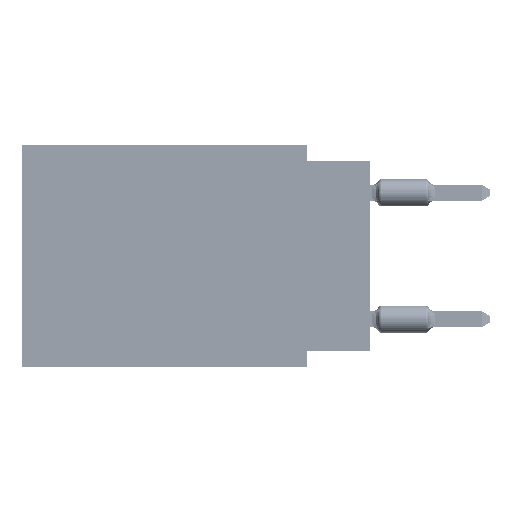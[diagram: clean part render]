
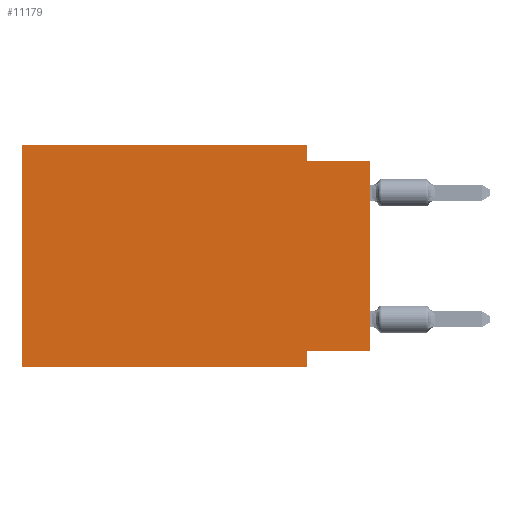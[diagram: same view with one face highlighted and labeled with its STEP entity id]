
A CAD part, left-side view. The second image highlights one B-rep face of the part: STEP entity #11179.
In plain terms, the highlighted planar face has unit normal (-1, 0, 0).
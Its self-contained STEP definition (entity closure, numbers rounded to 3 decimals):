
#1125 = CARTESIAN_POINT ( 'NONE',  ( 0., 0., -8.255 ) ) ;
#1972 = LINE ( 'NONE', #7984, #21266 ) ;
#5034 = EDGE_CURVE ( 'NONE', #32759, #79217, #30150, .T. ) ;
#5221 = CARTESIAN_POINT ( 'NONE',  ( 0., 2.54, 0. ) ) ;
#5799 = DIRECTION ( 'NONE',  ( 0., 0., 1. ) ) ;
#7984 = CARTESIAN_POINT ( 'NONE',  ( 0., 2.54, 0. ) ) ;
#10133 = VECTOR ( 'NONE', #76209, 1000. ) ;
#11179 = ADVANCED_FACE ( 'NONE', ( #45093 ), #71273, .F. ) ;
#11938 = CARTESIAN_POINT ( 'NONE',  ( 0., 0., -0.635 ) ) ;
#12740 = DIRECTION ( 'NONE',  ( 0., 1., 0. ) ) ;
#12816 = DIRECTION ( 'NONE',  ( 0., -1., 0. ) ) ;
#16610 = EDGE_CURVE ( 'NONE', #21372, #56353, #16953, .T. ) ;
#16953 = LINE ( 'NONE', #37131, #10133 ) ;
#17264 = DIRECTION ( 'NONE',  ( 0., -1., 0. ) ) ;
#17444 = CARTESIAN_POINT ( 'NONE',  ( 0., 13.97, 0. ) ) ;
#17733 = EDGE_CURVE ( 'NONE', #38163, #23053, #1972, .T. ) ;
#18718 = LINE ( 'NONE', #17444, #49562 ) ;
#21266 = VECTOR ( 'NONE', #40644, 1000. ) ;
#21372 = VERTEX_POINT ( 'NONE', #33781 ) ;
#23053 = VERTEX_POINT ( 'NONE', #28946 ) ;
#26891 = ORIENTED_EDGE ( 'NONE', *, *, #17733, .F. ) ;
#28946 = CARTESIAN_POINT ( 'NONE',  ( 0., 2.54, -0.635 ) ) ;
#29073 = ORIENTED_EDGE ( 'NONE', *, *, #5034, .T. ) ;
#29347 = AXIS2_PLACEMENT_3D ( 'NONE', #34309, #33896, #41602 ) ;
#29503 = EDGE_LOOP ( 'NONE', ( #34919, #46568, #26891, #70943, #56442, #29073, #61359, #41374 ) ) ;
#30150 = LINE ( 'NONE', #31843, #45351 ) ;
#30372 = EDGE_CURVE ( 'NONE', #21372, #83384, #59988, .T. ) ;
#31843 = CARTESIAN_POINT ( 'NONE',  ( 0., 13.97, -8.89 ) ) ;
#32759 = VERTEX_POINT ( 'NONE', #78496 ) ;
#33781 = CARTESIAN_POINT ( 'NONE',  ( 0., 0., -8.255 ) ) ;
#33896 = DIRECTION ( 'NONE',  ( 1., 0., 0. ) ) ;
#34309 = CARTESIAN_POINT ( 'NONE',  ( 0., 13.97, 0. ) ) ;
#34633 = VERTEX_POINT ( 'NONE', #61239 ) ;
#34919 = ORIENTED_EDGE ( 'NONE', *, *, #16610, .T. ) ;
#37131 = CARTESIAN_POINT ( 'NONE',  ( 0., 0., 0. ) ) ;
#38163 = VERTEX_POINT ( 'NONE', #5221 ) ;
#40644 = DIRECTION ( 'NONE',  ( 0., 0., -1. ) ) ;
#41374 = ORIENTED_EDGE ( 'NONE', *, *, #30372, .F. ) ;
#41602 = DIRECTION ( 'NONE',  ( 0., 0., -1. ) ) ;
#45093 = FACE_OUTER_BOUND ( 'NONE', #29503, .T. ) ;
#45116 = CARTESIAN_POINT ( 'NONE',  ( 0., 2.54, -8.89 ) ) ;
#45167 = VECTOR ( 'NONE', #12740, 1000. ) ;
#45351 = VECTOR ( 'NONE', #17264, 1000. ) ;
#46568 = ORIENTED_EDGE ( 'NONE', *, *, #63101, .F. ) ;
#49562 = VECTOR ( 'NONE', #5799, 1000. ) ;
#49783 = VECTOR ( 'NONE', #69328, 1000. ) ;
#51070 = CARTESIAN_POINT ( 'NONE',  ( 0., 0., -0.635 ) ) ;
#52403 = EDGE_CURVE ( 'NONE', #32759, #34633, #18718, .T. ) ;
#55951 = EDGE_CURVE ( 'NONE', #83384, #79217, #77733, .T. ) ;
#56353 = VERTEX_POINT ( 'NONE', #11938 ) ;
#56442 = ORIENTED_EDGE ( 'NONE', *, *, #52403, .F. ) ;
#59988 = LINE ( 'NONE', #1125, #45167 ) ;
#61239 = CARTESIAN_POINT ( 'NONE',  ( 0., 13.97, 0. ) ) ;
#61359 = ORIENTED_EDGE ( 'NONE', *, *, #55951, .F. ) ;
#62179 = EDGE_CURVE ( 'NONE', #34633, #38163, #69755, .T. ) ;
#63101 = EDGE_CURVE ( 'NONE', #23053, #56353, #84559, .T. ) ;
#64912 = VECTOR ( 'NONE', #12816, 1000. ) ;
#69328 = DIRECTION ( 'NONE',  ( 0., -1., 0. ) ) ;
#69755 = LINE ( 'NONE', #70164, #49783 ) ;
#70164 = CARTESIAN_POINT ( 'NONE',  ( 0., 13.97, 0. ) ) ;
#70920 = CARTESIAN_POINT ( 'NONE',  ( 0., 2.54, -8.255 ) ) ;
#70943 = ORIENTED_EDGE ( 'NONE', *, *, #62179, .F. ) ;
#71133 = VECTOR ( 'NONE', #71295, 1000. ) ;
#71273 = PLANE ( 'NONE',  #29347 ) ;
#71295 = DIRECTION ( 'NONE',  ( 0., 0., -1. ) ) ;
#76209 = DIRECTION ( 'NONE',  ( 0., 0., 1. ) ) ;
#77733 = LINE ( 'NONE', #45116, #71133 ) ;
#78496 = CARTESIAN_POINT ( 'NONE',  ( 0., 13.97, -8.89 ) ) ;
#79217 = VERTEX_POINT ( 'NONE', #83255 ) ;
#83255 = CARTESIAN_POINT ( 'NONE',  ( 0., 2.54, -8.89 ) ) ;
#83384 = VERTEX_POINT ( 'NONE', #70920 ) ;
#84559 = LINE ( 'NONE', #51070, #64912 ) ;
